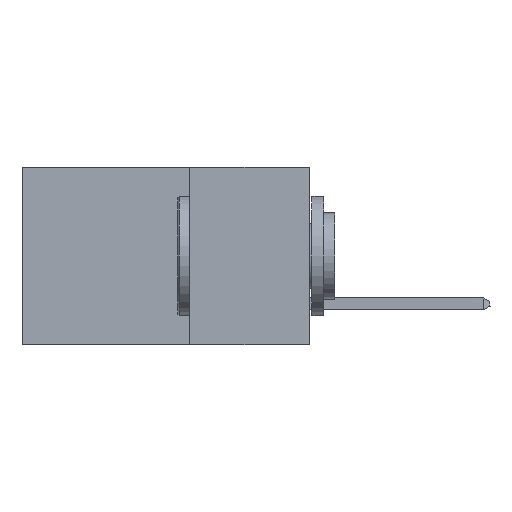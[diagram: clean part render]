
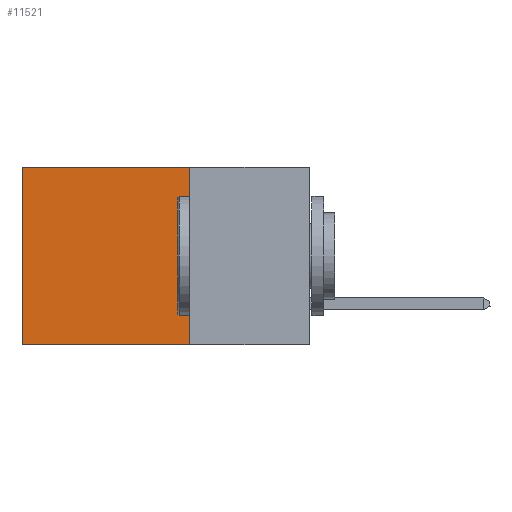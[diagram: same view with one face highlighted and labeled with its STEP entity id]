
A CAD part, left-side view. The second image highlights one B-rep face of the part: STEP entity #11521.
In plain terms, the highlighted planar face has unit normal (-1, 0, 0).
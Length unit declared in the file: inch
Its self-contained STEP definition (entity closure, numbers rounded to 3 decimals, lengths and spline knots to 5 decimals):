
#659 = LINE ( 'NONE', #5700, #5946 ) ;
#1499 = VERTEX_POINT ( 'NONE', #12416 ) ;
#1722 = PLANE ( 'NONE',  #5195 ) ;
#1782 = CARTESIAN_POINT ( 'NONE',  ( 0.2875, 0.25, 0. ) ) ;
#3138 = DIRECTION ( 'NONE',  ( 0., 0., -1. ) ) ;
#3705 = EDGE_CURVE ( 'NONE', #17242, #16122, #15888, .T. ) ;
#3736 = ORIENTED_EDGE ( 'NONE', *, *, #12834, .T. ) ;
#4423 = DIRECTION ( 'NONE',  ( 1., 0., 0. ) ) ;
#4991 = DIRECTION ( 'NONE',  ( 0., 0., -1. ) ) ;
#5113 = CARTESIAN_POINT ( 'NONE',  ( 0.2875, 0.25, -0.37 ) ) ;
#5195 = AXIS2_PLACEMENT_3D ( 'NONE', #1782, #4423, #3138 ) ;
#5700 = CARTESIAN_POINT ( 'NONE',  ( 0.2875, 0.25, -0.37 ) ) ;
#5809 = LINE ( 'NONE', #8406, #10727 ) ;
#5946 = VECTOR ( 'NONE', #14409, 39.37008 ) ;
#6016 = DIRECTION ( 'NONE',  ( 0., 0., -1. ) ) ;
#7452 = VECTOR ( 'NONE', #4991, 39.37008 ) ;
#8406 = CARTESIAN_POINT ( 'NONE',  ( 0.2875, 0.25, 0. ) ) ;
#8924 = ORIENTED_EDGE ( 'NONE', *, *, #16770, .T. ) ;
#9112 = VECTOR ( 'NONE', #6016, 39.37008 ) ;
#10105 = ORIENTED_EDGE ( 'NONE', *, *, #3705, .F. ) ;
#10404 = CARTESIAN_POINT ( 'NONE',  ( 0.2875, 0.25, 0. ) ) ;
#10727 = VECTOR ( 'NONE', #18788, 39.37008 ) ;
#11284 = CARTESIAN_POINT ( 'NONE',  ( 0.2875, 0.25, 0. ) ) ;
#11521 = ADVANCED_FACE ( 'NONE', ( #15014 ), #1722, .F. ) ;
#12012 = EDGE_LOOP ( 'NONE', ( #8924, #18852, #10105, #3736 ) ) ;
#12416 = CARTESIAN_POINT ( 'NONE',  ( 0.2875, 0.6, -0.37 ) ) ;
#12834 = EDGE_CURVE ( 'NONE', #17242, #14709, #5809, .T. ) ;
#13952 = CARTESIAN_POINT ( 'NONE',  ( 0.2875, 0.6, 0. ) ) ;
#14409 = DIRECTION ( 'NONE',  ( 0., 1., 0. ) ) ;
#14709 = VERTEX_POINT ( 'NONE', #15479 ) ;
#15014 = FACE_OUTER_BOUND ( 'NONE', #12012, .T. ) ;
#15445 = LINE ( 'NONE', #13952, #7452 ) ;
#15479 = CARTESIAN_POINT ( 'NONE',  ( 0.2875, 0.6, 0. ) ) ;
#15888 = LINE ( 'NONE', #10404, #9112 ) ;
#16122 = VERTEX_POINT ( 'NONE', #5113 ) ;
#16770 = EDGE_CURVE ( 'NONE', #14709, #1499, #15445, .T. ) ;
#17242 = VERTEX_POINT ( 'NONE', #11284 ) ;
#18788 = DIRECTION ( 'NONE',  ( 0., 1., 0. ) ) ;
#18852 = ORIENTED_EDGE ( 'NONE', *, *, #18977, .F. ) ;
#18977 = EDGE_CURVE ( 'NONE', #16122, #1499, #659, .T. ) ;
